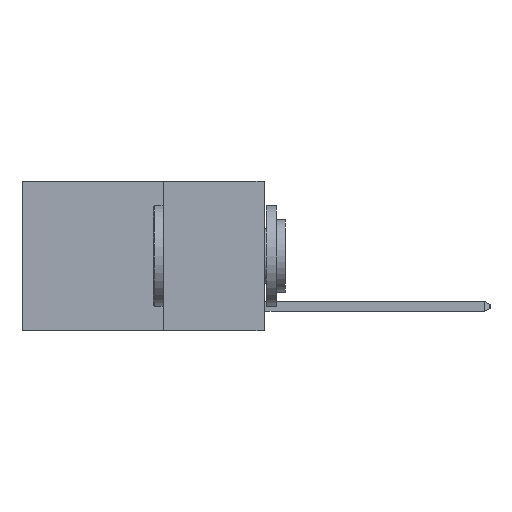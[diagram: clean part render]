
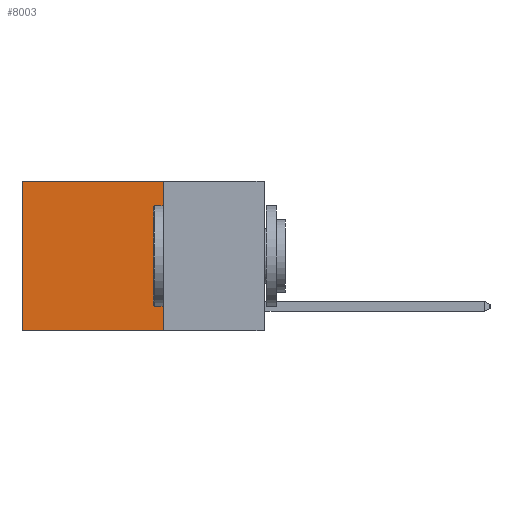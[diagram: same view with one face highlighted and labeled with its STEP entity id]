
A CAD part, left-side view. The second image highlights one B-rep face of the part: STEP entity #8003.
In plain terms, the highlighted planar face has unit normal (-1, 0, 0).
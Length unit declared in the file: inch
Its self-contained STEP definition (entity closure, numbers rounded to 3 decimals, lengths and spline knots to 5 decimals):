
#154 = CARTESIAN_POINT ( 'NONE',  ( 0.2625, 0.25, -0.37 ) ) ;
#814 = CARTESIAN_POINT ( 'NONE',  ( 0.2625, 0.6, 0. ) ) ;
#931 = DIRECTION ( 'NONE',  ( 0., 1., 0. ) ) ;
#961 = EDGE_CURVE ( 'NONE', #1417, #3154, #6905, .T. ) ;
#1417 = VERTEX_POINT ( 'NONE', #6539 ) ;
#1450 = DIRECTION ( 'NONE',  ( 0., 1., 0. ) ) ;
#1510 = EDGE_LOOP ( 'NONE', ( #6919, #6944, #6997, #7059 ) ) ;
#1512 = CARTESIAN_POINT ( 'NONE',  ( 0.2625, 0.25, 0. ) ) ;
#1651 = CARTESIAN_POINT ( 'NONE',  ( 0.2625, 0.6, 0. ) ) ;
#2055 = PLANE ( 'NONE',  #6441 ) ;
#2804 = DIRECTION ( 'NONE',  ( 1., 0., 0. ) ) ;
#2834 = LINE ( 'NONE', #7714, #7106 ) ;
#2857 = VECTOR ( 'NONE', #1450, 39.37008 ) ;
#3154 = VERTEX_POINT ( 'NONE', #814 ) ;
#3345 = VERTEX_POINT ( 'NONE', #6305 ) ;
#3899 = EDGE_CURVE ( 'NONE', #3154, #8707, #5044, .T. ) ;
#5044 = LINE ( 'NONE', #1651, #8819 ) ;
#5086 = LINE ( 'NONE', #154, #8862 ) ;
#5109 = CARTESIAN_POINT ( 'NONE',  ( 0.2625, 0.6, -0.37 ) ) ;
#6156 = DIRECTION ( 'NONE',  ( 0., 0., -1. ) ) ;
#6187 = DIRECTION ( 'NONE',  ( 0., 0., -1. ) ) ;
#6305 = CARTESIAN_POINT ( 'NONE',  ( 0.2625, 0.25, -0.37 ) ) ;
#6441 = AXIS2_PLACEMENT_3D ( 'NONE', #7358, #2804, #8107 ) ;
#6539 = CARTESIAN_POINT ( 'NONE',  ( 0.2625, 0.25, 0. ) ) ;
#6905 = LINE ( 'NONE', #1512, #2857 ) ;
#6919 = ORIENTED_EDGE ( 'NONE', *, *, #3899, .T. ) ;
#6944 = ORIENTED_EDGE ( 'NONE', *, *, #7194, .F. ) ;
#6997 = ORIENTED_EDGE ( 'NONE', *, *, #7208, .F. ) ;
#7059 = ORIENTED_EDGE ( 'NONE', *, *, #961, .T. ) ;
#7106 = VECTOR ( 'NONE', #6187, 39.37008 ) ;
#7194 = EDGE_CURVE ( 'NONE', #3345, #8707, #5086, .T. ) ;
#7208 = EDGE_CURVE ( 'NONE', #1417, #3345, #2834, .T. ) ;
#7358 = CARTESIAN_POINT ( 'NONE',  ( 0.2625, 0.25, 0. ) ) ;
#7575 = FACE_OUTER_BOUND ( 'NONE', #1510, .T. ) ;
#7714 = CARTESIAN_POINT ( 'NONE',  ( 0.2625, 0.25, 0. ) ) ;
#8003 = ADVANCED_FACE ( 'NONE', ( #7575 ), #2055, .F. ) ;
#8107 = DIRECTION ( 'NONE',  ( 0., 0., -1. ) ) ;
#8707 = VERTEX_POINT ( 'NONE', #5109 ) ;
#8819 = VECTOR ( 'NONE', #6156, 39.37008 ) ;
#8862 = VECTOR ( 'NONE', #931, 39.37008 ) ;
